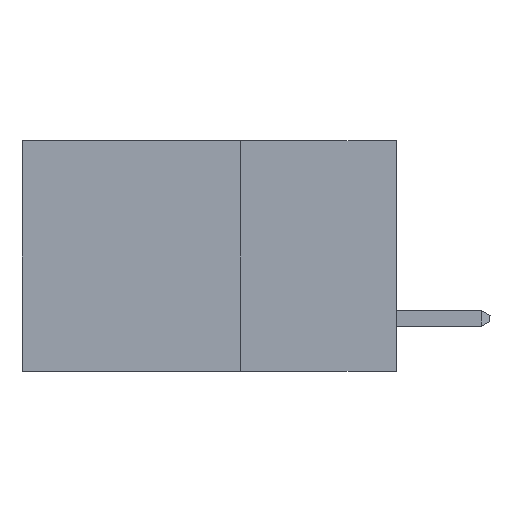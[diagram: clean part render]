
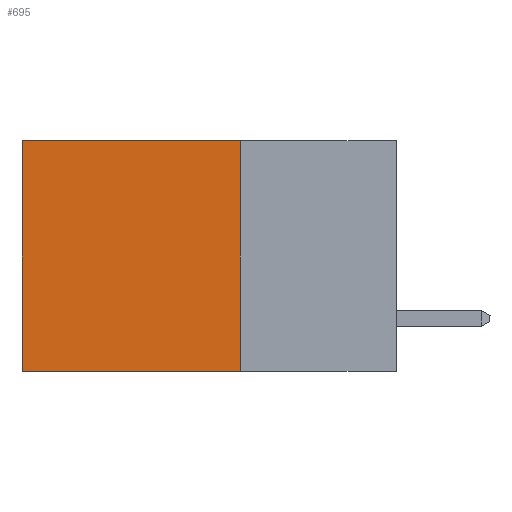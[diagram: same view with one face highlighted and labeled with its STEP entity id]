
A CAD part, left-side view. The second image highlights one B-rep face of the part: STEP entity #695.
In plain terms, the highlighted planar face has unit normal (-1, 0, 0).
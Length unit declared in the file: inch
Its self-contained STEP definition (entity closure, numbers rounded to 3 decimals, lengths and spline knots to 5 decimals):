
#66 = VERTEX_POINT ( 'NONE', #10013 ) ;
#206 = EDGE_CURVE ( 'NONE', #1512, #6587, #4951, .T. ) ;
#479 = DIRECTION ( 'NONE',  ( 0., 0., -1. ) ) ;
#695 = ADVANCED_FACE ( 'NONE', ( #6270 ), #12328, .F. ) ;
#1393 = EDGE_LOOP ( 'NONE', ( #11979, #2630, #3775, #6581 ) ) ;
#1512 = VERTEX_POINT ( 'NONE', #2705 ) ;
#2630 = ORIENTED_EDGE ( 'NONE', *, *, #7933, .F. ) ;
#2705 = CARTESIAN_POINT ( 'NONE',  ( 0.2615, 0.25, 0. ) ) ;
#3091 = VECTOR ( 'NONE', #479, 39.37008 ) ;
#3759 = DIRECTION ( 'NONE',  ( 0., 1., 0. ) ) ;
#3775 = ORIENTED_EDGE ( 'NONE', *, *, #206, .F. ) ;
#4518 = CARTESIAN_POINT ( 'NONE',  ( 0.2615, 0.6, -0.37 ) ) ;
#4845 = LINE ( 'NONE', #8937, #7391 ) ;
#4951 = LINE ( 'NONE', #11131, #9454 ) ;
#5303 = VERTEX_POINT ( 'NONE', #5851 ) ;
#5836 = DIRECTION ( 'NONE',  ( 0., 1., 0. ) ) ;
#5851 = CARTESIAN_POINT ( 'NONE',  ( 0.2615, 0.6, -0.37 ) ) ;
#5928 = CARTESIAN_POINT ( 'NONE',  ( 0.2615, 0.25, -0.37 ) ) ;
#6270 = FACE_OUTER_BOUND ( 'NONE', #1393, .T. ) ;
#6581 = ORIENTED_EDGE ( 'NONE', *, *, #12020, .T. ) ;
#6587 = VERTEX_POINT ( 'NONE', #5928 ) ;
#7362 = DIRECTION ( 'NONE',  ( 0., 0., -1. ) ) ;
#7391 = VECTOR ( 'NONE', #3759, 39.37008 ) ;
#7933 = EDGE_CURVE ( 'NONE', #6587, #5303, #4845, .T. ) ;
#8937 = CARTESIAN_POINT ( 'NONE',  ( 0.2615, 0.25, -0.37 ) ) ;
#9060 = CARTESIAN_POINT ( 'NONE',  ( 0.2615, 0.25, 0. ) ) ;
#9368 = CARTESIAN_POINT ( 'NONE',  ( 0.2615, 0.25, -0.37 ) ) ;
#9454 = VECTOR ( 'NONE', #11209, 39.37008 ) ;
#9695 = AXIS2_PLACEMENT_3D ( 'NONE', #9368, #10385, #7362 ) ;
#9716 = LINE ( 'NONE', #4518, #3091 ) ;
#9749 = EDGE_CURVE ( 'NONE', #66, #5303, #9716, .T. ) ;
#10013 = CARTESIAN_POINT ( 'NONE',  ( 0.2615, 0.6, 0. ) ) ;
#10158 = LINE ( 'NONE', #9060, #11808 ) ;
#10385 = DIRECTION ( 'NONE',  ( 1., 0., 0. ) ) ;
#11131 = CARTESIAN_POINT ( 'NONE',  ( 0.2615, 0.25, -0.37 ) ) ;
#11209 = DIRECTION ( 'NONE',  ( 0., 0., -1. ) ) ;
#11808 = VECTOR ( 'NONE', #5836, 39.37008 ) ;
#11979 = ORIENTED_EDGE ( 'NONE', *, *, #9749, .T. ) ;
#12020 = EDGE_CURVE ( 'NONE', #1512, #66, #10158, .T. ) ;
#12328 = PLANE ( 'NONE',  #9695 ) ;
